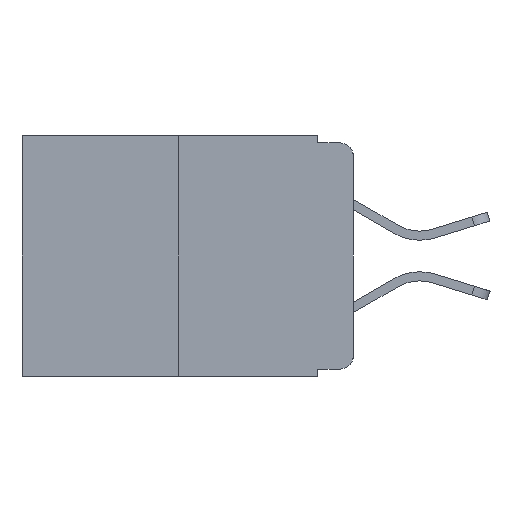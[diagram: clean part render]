
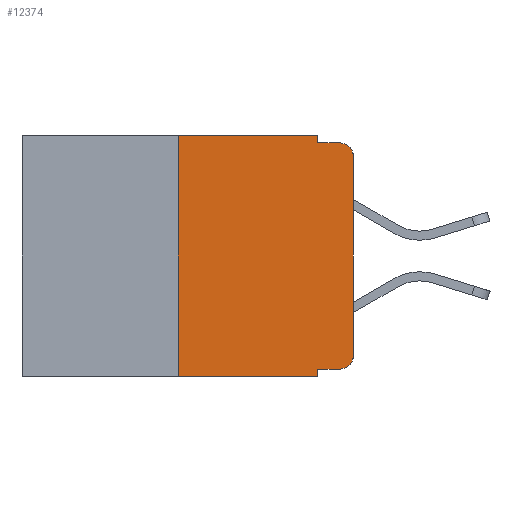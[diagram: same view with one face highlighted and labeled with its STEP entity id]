
A CAD part, left-side view. The second image highlights one B-rep face of the part: STEP entity #12374.
In plain terms, the highlighted planar face has unit normal (-1, 0, 0).
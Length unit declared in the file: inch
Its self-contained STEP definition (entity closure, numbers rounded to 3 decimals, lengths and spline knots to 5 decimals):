
#29 = EDGE_LOOP ( 'NONE', ( #4481, #12523, #1641, #1165, #12143, #10208, #8097, #325, #8790, #6043 ) ) ;
#278 = CARTESIAN_POINT ( 'NONE',  ( 0., 0., -0.313 ) ) ;
#325 = ORIENTED_EDGE ( 'NONE', *, *, #5467, .F. ) ;
#528 = CARTESIAN_POINT ( 'NONE',  ( 0., 0., -0.03 ) ) ;
#774 = VECTOR ( 'NONE', #9757, 39.37008 ) ;
#814 = CARTESIAN_POINT ( 'NONE',  ( 0., 0.051, -0.333 ) ) ;
#1139 = CARTESIAN_POINT ( 'NONE',  ( 0., 0.051, -0.01 ) ) ;
#1161 = VECTOR ( 'NONE', #11178, 39.37008 ) ;
#1165 = ORIENTED_EDGE ( 'NONE', *, *, #11104, .F. ) ;
#1268 = DIRECTION ( 'NONE',  ( -1., 0., 0. ) ) ;
#1439 = CARTESIAN_POINT ( 'NONE',  ( 0., 0.051, 0. ) ) ;
#1640 = CARTESIAN_POINT ( 'NONE',  ( 0., 0.02, -0.03 ) ) ;
#1641 = ORIENTED_EDGE ( 'NONE', *, *, #11062, .F. ) ;
#1646 = EDGE_CURVE ( 'NONE', #1841, #8167, #3002, .T. ) ;
#1841 = VERTEX_POINT ( 'NONE', #10467 ) ;
#2110 = LINE ( 'NONE', #11948, #4424 ) ;
#2121 = CARTESIAN_POINT ( 'NONE',  ( 0., 0.473, 0. ) ) ;
#2131 = DIRECTION ( 'NONE',  ( 0., -1., 0. ) ) ;
#2167 = CARTESIAN_POINT ( 'NONE',  ( 0., 0.02, -0.333 ) ) ;
#2260 = LINE ( 'NONE', #10748, #8206 ) ;
#2420 = DIRECTION ( 'NONE',  ( 0., 0., -1. ) ) ;
#2525 = VECTOR ( 'NONE', #2420, 39.37008 ) ;
#2628 = DIRECTION ( 'NONE',  ( 0., -1., 0. ) ) ;
#2727 = CARTESIAN_POINT ( 'NONE',  ( 0., 0.473, 0. ) ) ;
#2782 = VECTOR ( 'NONE', #4789, 39.37008 ) ;
#3002 = LINE ( 'NONE', #9209, #1161 ) ;
#3078 = DIRECTION ( 'NONE',  ( 1., 0., 0. ) ) ;
#3133 = EDGE_CURVE ( 'NONE', #1841, #10275, #10028, .T. ) ;
#3233 = VERTEX_POINT ( 'NONE', #528 ) ;
#3521 = AXIS2_PLACEMENT_3D ( 'NONE', #2121, #3078, #11791 ) ;
#3545 = DIRECTION ( 'NONE',  ( 0., 0., -1. ) ) ;
#3561 = EDGE_CURVE ( 'NONE', #10060, #12287, #2110, .T. ) ;
#4086 = LINE ( 'NONE', #1439, #2525 ) ;
#4424 = VECTOR ( 'NONE', #6220, 39.37008 ) ;
#4481 = ORIENTED_EDGE ( 'NONE', *, *, #7673, .T. ) ;
#4539 = CARTESIAN_POINT ( 'NONE',  ( 0., 0.051, 0. ) ) ;
#4625 = CARTESIAN_POINT ( 'NONE',  ( 0., 0.02, -0.01 ) ) ;
#4708 = FACE_OUTER_BOUND ( 'NONE', #29, .T. ) ;
#4789 = DIRECTION ( 'NONE',  ( 0., 0., 1. ) ) ;
#4917 = VERTEX_POINT ( 'NONE', #4625 ) ;
#4986 = CIRCLE ( 'NONE', #6415, 0.02 ) ;
#5095 = PLANE ( 'NONE',  #3521 ) ;
#5467 = EDGE_CURVE ( 'NONE', #10060, #10275, #4086, .T. ) ;
#5854 = LINE ( 'NONE', #10582, #2782 ) ;
#6043 = ORIENTED_EDGE ( 'NONE', *, *, #6076, .T. ) ;
#6055 = CARTESIAN_POINT ( 'NONE',  ( 0., 0.473, -0.343 ) ) ;
#6076 = EDGE_CURVE ( 'NONE', #12287, #11958, #4986, .T. ) ;
#6220 = DIRECTION ( 'NONE',  ( 0., -1., 0. ) ) ;
#6415 = AXIS2_PLACEMENT_3D ( 'NONE', #12077, #1268, #10020 ) ;
#6441 = LINE ( 'NONE', #2727, #11286 ) ;
#6844 = DIRECTION ( 'NONE',  ( 0., 0., -1. ) ) ;
#7520 = EDGE_CURVE ( 'NONE', #3233, #4917, #11925, .T. ) ;
#7673 = EDGE_CURVE ( 'NONE', #11958, #3233, #5854, .T. ) ;
#8097 = ORIENTED_EDGE ( 'NONE', *, *, #3133, .T. ) ;
#8167 = VERTEX_POINT ( 'NONE', #11352 ) ;
#8206 = VECTOR ( 'NONE', #6844, 39.37008 ) ;
#8365 = DIRECTION ( 'NONE',  ( -1., 0., 0. ) ) ;
#8790 = ORIENTED_EDGE ( 'NONE', *, *, #3561, .T. ) ;
#8871 = CARTESIAN_POINT ( 'NONE',  ( 0., 0.051, -0.343 ) ) ;
#9080 = AXIS2_PLACEMENT_3D ( 'NONE', #1640, #8365, #3545 ) ;
#9209 = CARTESIAN_POINT ( 'NONE',  ( 0., 0.25, 0. ) ) ;
#9757 = DIRECTION ( 'NONE',  ( 0., -1., 0. ) ) ;
#9889 = EDGE_CURVE ( 'NONE', #8167, #12085, #6441, .T. ) ;
#10020 = DIRECTION ( 'NONE',  ( 0., 0., -1. ) ) ;
#10028 = LINE ( 'NONE', #6055, #11579 ) ;
#10060 = VERTEX_POINT ( 'NONE', #814 ) ;
#10208 = ORIENTED_EDGE ( 'NONE', *, *, #1646, .F. ) ;
#10275 = VERTEX_POINT ( 'NONE', #8871 ) ;
#10286 = VERTEX_POINT ( 'NONE', #1139 ) ;
#10467 = CARTESIAN_POINT ( 'NONE',  ( 0., 0.25, -0.343 ) ) ;
#10582 = CARTESIAN_POINT ( 'NONE',  ( 0., 0., 0. ) ) ;
#10705 = CARTESIAN_POINT ( 'NONE',  ( 0., 0.051, -0.01 ) ) ;
#10748 = CARTESIAN_POINT ( 'NONE',  ( 0., 0.051, 0. ) ) ;
#11062 = EDGE_CURVE ( 'NONE', #10286, #4917, #11255, .T. ) ;
#11104 = EDGE_CURVE ( 'NONE', #12085, #10286, #2260, .T. ) ;
#11178 = DIRECTION ( 'NONE',  ( 0., 0., 1. ) ) ;
#11255 = LINE ( 'NONE', #10705, #774 ) ;
#11286 = VECTOR ( 'NONE', #2628, 39.37008 ) ;
#11352 = CARTESIAN_POINT ( 'NONE',  ( 0., 0.25, 0. ) ) ;
#11579 = VECTOR ( 'NONE', #2131, 39.37008 ) ;
#11791 = DIRECTION ( 'NONE',  ( 0., 0., -1. ) ) ;
#11925 = CIRCLE ( 'NONE', #9080, 0.02 ) ;
#11948 = CARTESIAN_POINT ( 'NONE',  ( 0., 0.051, -0.333 ) ) ;
#11958 = VERTEX_POINT ( 'NONE', #278 ) ;
#12077 = CARTESIAN_POINT ( 'NONE',  ( 0., 0.02, -0.313 ) ) ;
#12085 = VERTEX_POINT ( 'NONE', #4539 ) ;
#12143 = ORIENTED_EDGE ( 'NONE', *, *, #9889, .F. ) ;
#12287 = VERTEX_POINT ( 'NONE', #2167 ) ;
#12374 = ADVANCED_FACE ( 'NONE', ( #4708 ), #5095, .F. ) ;
#12523 = ORIENTED_EDGE ( 'NONE', *, *, #7520, .T. ) ;
